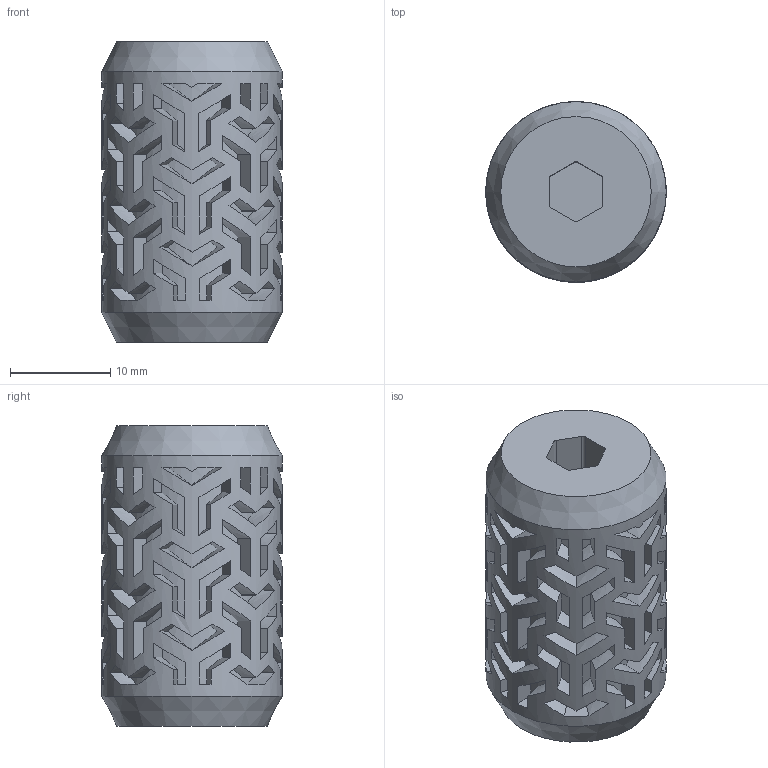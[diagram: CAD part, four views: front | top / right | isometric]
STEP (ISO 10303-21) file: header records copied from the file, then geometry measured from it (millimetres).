
FILE_DESCRIPTION(/* description */ (''),/* implementation_level */ '2;1');
FILE_NAME(/* name */ 'Charging Handle.step',/* time_stamp */ '2022-05-11T21:18:21-06:00',/* author */ (''),/* organization */ (''),/* preprocessor_version */ 'ST-DEVELOPER v18.1',/* originating_system */ 'Autodesk Translation Framework v10.10.0.1391',/* authorisation */ '');
FILE_SCHEMA (('AUTOMOTIVE_DESIGN { 1 0 10303 214 3 1 1 }'));
Length unit declared in the file: millimetre
Products named in the file (1): Charging handle tri stip edition
Bounding box: 18 x 18 x 30 mm (x, y, z)
Volume: 6034.8 mm3; surface area: 4218.6 mm2
Topology: 1 solids, 1 shells, 534 faces, 1383 edges, 921 vertices
Faces by surface type: bspline 260, plane 193, cylinder 79, cone 2
Full cylindrical faces by diameter (mm): 18 x1
Entity records: 19772 total; most frequent: CARTESIAN_POINT 8431, ORIENTED_EDGE 2766, DIRECTION 1458, EDGE_CURVE 1383, VERTEX_POINT 921, LINE 762, VECTOR 762, EDGE_LOOP 604
